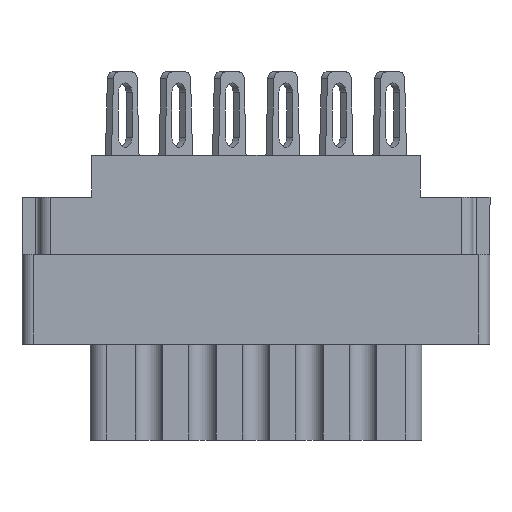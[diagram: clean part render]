
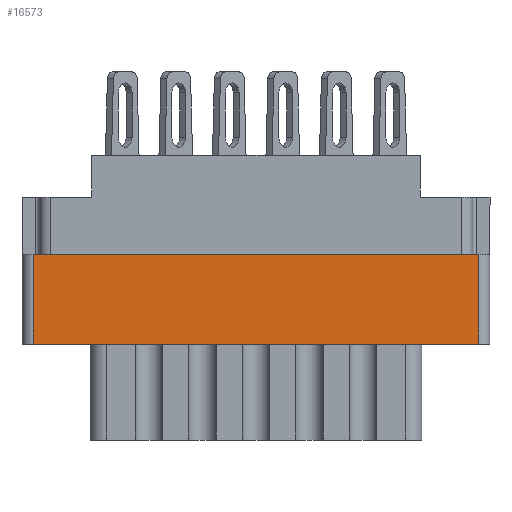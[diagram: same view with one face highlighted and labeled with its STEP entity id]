
A CAD part, front view. The second image highlights one B-rep face of the part: STEP entity #16573.
In plain terms, the highlighted planar face has unit normal (0, -1, 0).
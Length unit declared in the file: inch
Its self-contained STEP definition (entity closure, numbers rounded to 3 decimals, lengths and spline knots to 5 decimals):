
#708 = AXIS2_PLACEMENT_3D ( 'NONE', #17763, #8960, #5936 ) ;
#854 = VERTEX_POINT ( 'NONE', #13966 ) ;
#1039 = CARTESIAN_POINT ( 'NONE',  ( 0.624, -0.343, -0.529 ) ) ;
#1192 = EDGE_LOOP ( 'NONE', ( #15701, #15444, #9074, #16928 ) ) ;
#1425 = VERTEX_POINT ( 'NONE', #1039 ) ;
#1958 = VECTOR ( 'NONE', #10726, 39.37008 ) ;
#2140 = VECTOR ( 'NONE', #2731, 39.37008 ) ;
#2731 = DIRECTION ( 'NONE',  ( 0., 0., 1. ) ) ;
#2772 = CARTESIAN_POINT ( 'NONE',  ( 0.624, -0.343, -0.277 ) ) ;
#3070 = EDGE_CURVE ( 'NONE', #1425, #18875, #17881, .T. ) ;
#3312 = LINE ( 'NONE', #7404, #1958 ) ;
#4269 = EDGE_CURVE ( 'NONE', #854, #8386, #17225, .T. ) ;
#4914 = DIRECTION ( 'NONE',  ( 0., 0., 1. ) ) ;
#5936 = DIRECTION ( 'NONE',  ( 0., 0., -1. ) ) ;
#6323 = VECTOR ( 'NONE', #15573, 39.37008 ) ;
#6492 = CARTESIAN_POINT ( 'NONE',  ( 0.624, -0.343, -0.529 ) ) ;
#7404 = CARTESIAN_POINT ( 'NONE',  ( -0.656, -0.343, -0.277 ) ) ;
#8386 = VERTEX_POINT ( 'NONE', #9538 ) ;
#8960 = DIRECTION ( 'NONE',  ( 0., -1., 0. ) ) ;
#9074 = ORIENTED_EDGE ( 'NONE', *, *, #3070, .T. ) ;
#9465 = EDGE_CURVE ( 'NONE', #8386, #18875, #3312, .T. ) ;
#9538 = CARTESIAN_POINT ( 'NONE',  ( -0.624, -0.343, -0.277 ) ) ;
#9680 = CARTESIAN_POINT ( 'NONE',  ( -0.624, -0.343, -0.798 ) ) ;
#10726 = DIRECTION ( 'NONE',  ( 1., 0., 0. ) ) ;
#11083 = LINE ( 'NONE', #6492, #6323 ) ;
#11311 = FACE_OUTER_BOUND ( 'NONE', #1192, .T. ) ;
#11706 = CARTESIAN_POINT ( 'NONE',  ( 0.624, -0.343, -0.798 ) ) ;
#13966 = CARTESIAN_POINT ( 'NONE',  ( -0.624, -0.343, -0.529 ) ) ;
#15444 = ORIENTED_EDGE ( 'NONE', *, *, #18587, .F. ) ;
#15573 = DIRECTION ( 'NONE',  ( -1., 0., 0. ) ) ;
#15701 = ORIENTED_EDGE ( 'NONE', *, *, #4269, .F. ) ;
#16573 = ADVANCED_FACE ( 'NONE', ( #11311 ), #17286, .T. ) ;
#16928 = ORIENTED_EDGE ( 'NONE', *, *, #9465, .F. ) ;
#17225 = LINE ( 'NONE', #9680, #17445 ) ;
#17286 = PLANE ( 'NONE',  #708 ) ;
#17445 = VECTOR ( 'NONE', #4914, 39.37008 ) ;
#17763 = CARTESIAN_POINT ( 'NONE',  ( -0.624, -0.343, -0.798 ) ) ;
#17881 = LINE ( 'NONE', #11706, #2140 ) ;
#18587 = EDGE_CURVE ( 'NONE', #1425, #854, #11083, .T. ) ;
#18875 = VERTEX_POINT ( 'NONE', #2772 ) ;
